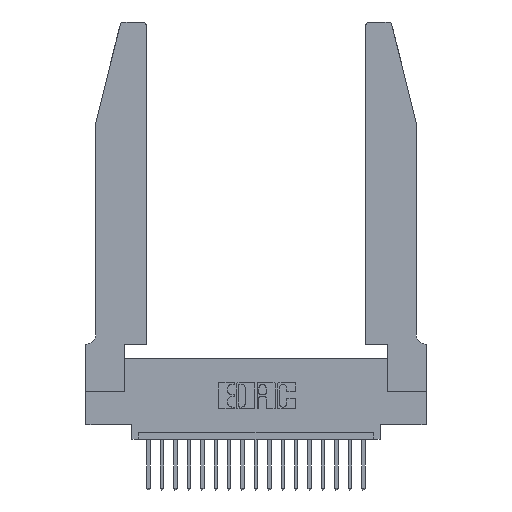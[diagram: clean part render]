
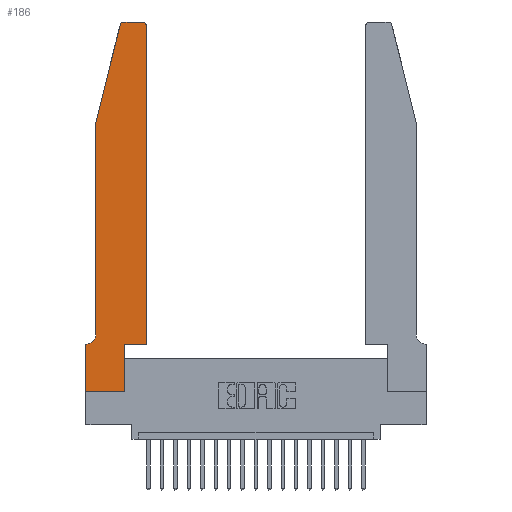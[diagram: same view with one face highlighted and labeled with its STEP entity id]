
A CAD part, top view. The second image highlights one B-rep face of the part: STEP entity #186.
In plain terms, the highlighted planar face has unit normal (0, 0, 1).
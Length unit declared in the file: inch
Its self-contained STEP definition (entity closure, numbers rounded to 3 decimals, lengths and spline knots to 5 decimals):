
#186 = ADVANCED_FACE ( 'NONE', ( #19307 ), #9597, .T. ) ;
#228 = VERTEX_POINT ( 'NONE', #14580 ) ;
#269 = LINE ( 'NONE', #4986, #13438 ) ;
#335 = AXIS2_PLACEMENT_3D ( 'NONE', #16507, #3460, #18140 ) ;
#394 = LINE ( 'NONE', #14529, #14850 ) ;
#416 = VERTEX_POINT ( 'NONE', #16554 ) ;
#826 = EDGE_CURVE ( 'NONE', #416, #19476, #269, .T. ) ;
#828 = ORIENTED_EDGE ( 'NONE', *, *, #1067, .T. ) ;
#1067 = EDGE_CURVE ( 'NONE', #5026, #8804, #5075, .T. ) ;
#1525 = AXIS2_PLACEMENT_3D ( 'NONE', #19672, #5079, #6610 ) ;
#1549 = ORIENTED_EDGE ( 'NONE', *, *, #8557, .T. ) ;
#1896 = DIRECTION ( 'NONE',  ( -0.239, -0.971, 0. ) ) ;
#2225 = VERTEX_POINT ( 'NONE', #16965 ) ;
#2435 = VECTOR ( 'NONE', #12841, 39.37008 ) ;
#2696 = CIRCLE ( 'NONE', #8349, 0.03 ) ;
#2784 = EDGE_CURVE ( 'NONE', #18144, #416, #18978, .T. ) ;
#2899 = CARTESIAN_POINT ( 'NONE',  ( 0.4205, 2.72, 0.37 ) ) ;
#3026 = CARTESIAN_POINT ( 'NONE',  ( 0.4505, 0.35, 0.37 ) ) ;
#3098 = CARTESIAN_POINT ( 'NONE',  ( 0.2865, 0.35, 0.37 ) ) ;
#3115 = CARTESIAN_POINT ( 'NONE',  ( 0.284, 2.72, 0.37 ) ) ;
#3388 = VERTEX_POINT ( 'NONE', #12910 ) ;
#3460 = DIRECTION ( 'NONE',  ( 0., 0., -1. ) ) ;
#4034 = LINE ( 'NONE', #8684, #5275 ) ;
#4041 = ORIENTED_EDGE ( 'NONE', *, *, #6918, .T. ) ;
#4068 = CARTESIAN_POINT ( 'NONE',  ( 0.0755, 2., 0.37 ) ) ;
#4851 = CIRCLE ( 'NONE', #335, 0.07 ) ;
#4962 = CARTESIAN_POINT ( 'NONE',  ( 0., 0., 0.37 ) ) ;
#4986 = CARTESIAN_POINT ( 'NONE',  ( 0.4505, 0.35, 0.37 ) ) ;
#5026 = VERTEX_POINT ( 'NONE', #11729 ) ;
#5075 = LINE ( 'NONE', #4068, #17498 ) ;
#5079 = DIRECTION ( 'NONE',  ( 0., 0., 1. ) ) ;
#5090 = ORIENTED_EDGE ( 'NONE', *, *, #15836, .T. ) ;
#5275 = VECTOR ( 'NONE', #16729, 39.37008 ) ;
#5382 = ORIENTED_EDGE ( 'NONE', *, *, #15074, .T. ) ;
#6155 = LINE ( 'NONE', #3026, #7168 ) ;
#6373 = ORIENTED_EDGE ( 'NONE', *, *, #11414, .T. ) ;
#6517 = CARTESIAN_POINT ( 'NONE',  ( 0.2865, 0., 0.37 ) ) ;
#6610 = DIRECTION ( 'NONE',  ( 1., 0., 0. ) ) ;
#6918 = EDGE_CURVE ( 'NONE', #9672, #13446, #12936, .T. ) ;
#7168 = VECTOR ( 'NONE', #14370, 39.37008 ) ;
#7228 = CARTESIAN_POINT ( 'NONE',  ( 0.0755, 0.42, 0.37 ) ) ;
#7713 = EDGE_CURVE ( 'NONE', #3388, #9672, #4034, .T. ) ;
#7733 = VECTOR ( 'NONE', #17382, 39.37008 ) ;
#8304 = DIRECTION ( 'NONE',  ( 1., 0., 0. ) ) ;
#8316 = CARTESIAN_POINT ( 'NONE',  ( 0.0755, 0.35, 0.37 ) ) ;
#8349 = AXIS2_PLACEMENT_3D ( 'NONE', #2899, #14252, #20565 ) ;
#8551 = ORIENTED_EDGE ( 'NONE', *, *, #7713, .T. ) ;
#8557 = EDGE_CURVE ( 'NONE', #228, #3388, #2696, .T. ) ;
#8684 = CARTESIAN_POINT ( 'NONE',  ( 0.2605, 2.75, 0.37 ) ) ;
#8804 = VERTEX_POINT ( 'NONE', #7228 ) ;
#9342 = ORIENTED_EDGE ( 'NONE', *, *, #15340, .T. ) ;
#9377 = EDGE_CURVE ( 'NONE', #19129, #2225, #14891, .T. ) ;
#9597 = PLANE ( 'NONE',  #1525 ) ;
#9672 = VERTEX_POINT ( 'NONE', #10198 ) ;
#9775 = LINE ( 'NONE', #8316, #7733 ) ;
#9851 = CARTESIAN_POINT ( 'NONE',  ( 0.25487, 2.72718, 0.37 ) ) ;
#10198 = CARTESIAN_POINT ( 'NONE',  ( 0.284, 2.75, 0.37 ) ) ;
#10428 = AXIS2_PLACEMENT_3D ( 'NONE', #3115, #11341, #14387 ) ;
#10519 = CARTESIAN_POINT ( 'NONE',  ( 0., 0., 0.37 ) ) ;
#10659 = DIRECTION ( 'NONE',  ( 1., 0., 0. ) ) ;
#11341 = DIRECTION ( 'NONE',  ( 0., 0., 1. ) ) ;
#11414 = EDGE_CURVE ( 'NONE', #19476, #228, #6155, .T. ) ;
#11729 = CARTESIAN_POINT ( 'NONE',  ( 0.0755, 2., 0.37 ) ) ;
#12160 = ORIENTED_EDGE ( 'NONE', *, *, #2784, .T. ) ;
#12214 = EDGE_CURVE ( 'NONE', #8804, #19007, #4851, .T. ) ;
#12274 = DIRECTION ( 'NONE',  ( 0., -1., 0. ) ) ;
#12385 = CARTESIAN_POINT ( 'NONE',  ( 0.0055, 0.35, 0.37 ) ) ;
#12596 = CARTESIAN_POINT ( 'NONE',  ( 0., 0.35, 0.37 ) ) ;
#12818 = DIRECTION ( 'NONE',  ( 0., 1., 0. ) ) ;
#12841 = DIRECTION ( 'NONE',  ( 0., -1., 0. ) ) ;
#12910 = CARTESIAN_POINT ( 'NONE',  ( 0.4205, 2.75, 0.37 ) ) ;
#12936 = CIRCLE ( 'NONE', #10428, 0.03 ) ;
#13438 = VECTOR ( 'NONE', #8304, 39.37008 ) ;
#13446 = VERTEX_POINT ( 'NONE', #9851 ) ;
#13611 = VECTOR ( 'NONE', #12818, 39.37008 ) ;
#14252 = DIRECTION ( 'NONE',  ( 0., 0., 1. ) ) ;
#14370 = DIRECTION ( 'NONE',  ( 0., 1., 0. ) ) ;
#14387 = DIRECTION ( 'NONE',  ( 1., 0., 0. ) ) ;
#14529 = CARTESIAN_POINT ( 'NONE',  ( 0.0755, 2., 0.37 ) ) ;
#14580 = CARTESIAN_POINT ( 'NONE',  ( 0.4505, 2.72, 0.37 ) ) ;
#14850 = VECTOR ( 'NONE', #1896, 39.37008 ) ;
#14891 = LINE ( 'NONE', #4962, #2435 ) ;
#15074 = EDGE_CURVE ( 'NONE', #19007, #19129, #9775, .T. ) ;
#15340 = EDGE_CURVE ( 'NONE', #2225, #18144, #19983, .T. ) ;
#15836 = EDGE_CURVE ( 'NONE', #13446, #5026, #394, .T. ) ;
#15970 = CARTESIAN_POINT ( 'NONE',  ( 0.4505, 0.35, 0.37 ) ) ;
#16476 = EDGE_LOOP ( 'NONE', ( #8551, #4041, #5090, #828, #20247, #5382, #17826, #9342, #12160, #18442, #6373, #1549 ) ) ;
#16507 = CARTESIAN_POINT ( 'NONE',  ( 0.0055, 0.42, 0.37 ) ) ;
#16554 = CARTESIAN_POINT ( 'NONE',  ( 0.2865, 0.35, 0.37 ) ) ;
#16729 = DIRECTION ( 'NONE',  ( -1., 0., 0. ) ) ;
#16965 = CARTESIAN_POINT ( 'NONE',  ( 0., 0., 0.37 ) ) ;
#17382 = DIRECTION ( 'NONE',  ( -1., 0., 0. ) ) ;
#17498 = VECTOR ( 'NONE', #12274, 39.37008 ) ;
#17826 = ORIENTED_EDGE ( 'NONE', *, *, #9377, .T. ) ;
#18140 = DIRECTION ( 'NONE',  ( -1., 0., 0. ) ) ;
#18144 = VERTEX_POINT ( 'NONE', #6517 ) ;
#18442 = ORIENTED_EDGE ( 'NONE', *, *, #826, .T. ) ;
#18705 = VECTOR ( 'NONE', #10659, 39.37008 ) ;
#18978 = LINE ( 'NONE', #3098, #13611 ) ;
#19007 = VERTEX_POINT ( 'NONE', #12385 ) ;
#19129 = VERTEX_POINT ( 'NONE', #12596 ) ;
#19307 = FACE_OUTER_BOUND ( 'NONE', #16476, .T. ) ;
#19476 = VERTEX_POINT ( 'NONE', #15970 ) ;
#19672 = CARTESIAN_POINT ( 'NONE',  ( 0., 0.35, 0.37 ) ) ;
#19983 = LINE ( 'NONE', #10519, #18705 ) ;
#20247 = ORIENTED_EDGE ( 'NONE', *, *, #12214, .T. ) ;
#20565 = DIRECTION ( 'NONE',  ( 1., 0., 0. ) ) ;
